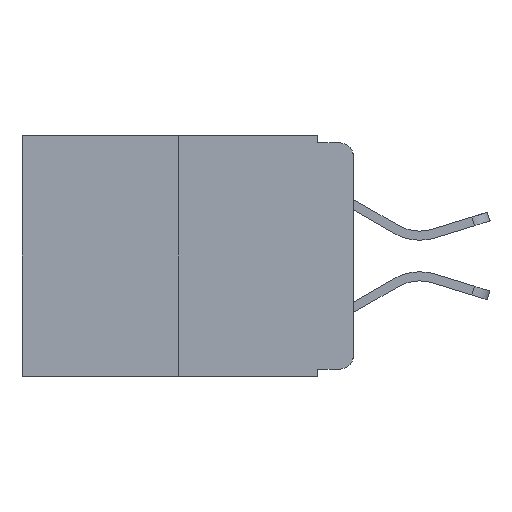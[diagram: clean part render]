
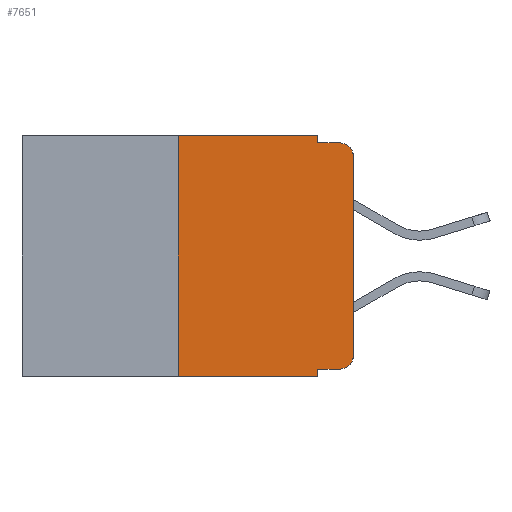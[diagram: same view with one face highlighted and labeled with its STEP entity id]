
A CAD part, left-side view. The second image highlights one B-rep face of the part: STEP entity #7651.
In plain terms, the highlighted planar face has unit normal (-1, 0, 0).
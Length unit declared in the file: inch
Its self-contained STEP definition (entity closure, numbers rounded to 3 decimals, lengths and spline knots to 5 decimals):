
#76 = CIRCLE ( 'NONE', #13283, 0.02 ) ;
#86 = ORIENTED_EDGE ( 'NONE', *, *, #2032, .F. ) ;
#299 = ORIENTED_EDGE ( 'NONE', *, *, #17580, .F. ) ;
#850 = DIRECTION ( 'NONE',  ( 1., 0., 0. ) ) ;
#975 = CARTESIAN_POINT ( 'NONE',  ( 0., 0.02, -0.03 ) ) ;
#1008 = EDGE_CURVE ( 'NONE', #21379, #19777, #14824, .T. ) ;
#1170 = VECTOR ( 'NONE', #16468, 39.37008 ) ;
#1306 = EDGE_CURVE ( 'NONE', #8760, #17799, #76, .T. ) ;
#1410 = CARTESIAN_POINT ( 'NONE',  ( 0., 0., 0. ) ) ;
#1425 = DIRECTION ( 'NONE',  ( 0., -1., 0. ) ) ;
#2007 = VECTOR ( 'NONE', #11165, 39.37008 ) ;
#2032 = EDGE_CURVE ( 'NONE', #8149, #3900, #17525, .T. ) ;
#2465 = CIRCLE ( 'NONE', #16862, 0.02 ) ;
#2495 = ORIENTED_EDGE ( 'NONE', *, *, #9484, .T. ) ;
#2614 = VERTEX_POINT ( 'NONE', #10916 ) ;
#2711 = DIRECTION ( 'NONE',  ( 0., 0., -1. ) ) ;
#3086 = FACE_OUTER_BOUND ( 'NONE', #14970, .T. ) ;
#3099 = VERTEX_POINT ( 'NONE', #3815 ) ;
#3127 = VECTOR ( 'NONE', #1425, 39.37008 ) ;
#3337 = VERTEX_POINT ( 'NONE', #9422 ) ;
#3755 = DIRECTION ( 'NONE',  ( 0., -1., 0. ) ) ;
#3815 = CARTESIAN_POINT ( 'NONE',  ( 0., 0.051, 0. ) ) ;
#3900 = VERTEX_POINT ( 'NONE', #13992 ) ;
#4194 = CARTESIAN_POINT ( 'NONE',  ( 0., 0.02, -0.333 ) ) ;
#4397 = VECTOR ( 'NONE', #12512, 39.37008 ) ;
#4543 = AXIS2_PLACEMENT_3D ( 'NONE', #11037, #850, #12675 ) ;
#4581 = CARTESIAN_POINT ( 'NONE',  ( 0., 0.051, -0.01 ) ) ;
#4670 = VERTEX_POINT ( 'NONE', #20590 ) ;
#4853 = DIRECTION ( 'NONE',  ( 0., 0., 1. ) ) ;
#5037 = CARTESIAN_POINT ( 'NONE',  ( 0., 0.25, 0. ) ) ;
#5074 = ORIENTED_EDGE ( 'NONE', *, *, #6944, .T. ) ;
#5251 = VECTOR ( 'NONE', #4853, 39.37008 ) ;
#5361 = CARTESIAN_POINT ( 'NONE',  ( 0., 0.051, -0.01 ) ) ;
#5389 = CARTESIAN_POINT ( 'NONE',  ( 0., 0.473, -0.343 ) ) ;
#6001 = CARTESIAN_POINT ( 'NONE',  ( 0., 0.051, 0. ) ) ;
#6297 = CARTESIAN_POINT ( 'NONE',  ( 0., 0.02, -0.313 ) ) ;
#6696 = CARTESIAN_POINT ( 'NONE',  ( 0., 0.473, 0. ) ) ;
#6736 = EDGE_CURVE ( 'NONE', #2614, #8760, #16357, .T. ) ;
#6944 = EDGE_CURVE ( 'NONE', #8149, #4670, #20298, .T. ) ;
#7066 = DIRECTION ( 'NONE',  ( -1., 0., 0. ) ) ;
#7651 = ADVANCED_FACE ( 'NONE', ( #3086 ), #17428, .F. ) ;
#7704 = EDGE_CURVE ( 'NONE', #2614, #4670, #11034, .T. ) ;
#8149 = VERTEX_POINT ( 'NONE', #12315 ) ;
#8176 = CARTESIAN_POINT ( 'NONE',  ( 0., 0.02, -0.01 ) ) ;
#8419 = EDGE_CURVE ( 'NONE', #3900, #3099, #14533, .T. ) ;
#8760 = VERTEX_POINT ( 'NONE', #4194 ) ;
#8970 = ORIENTED_EDGE ( 'NONE', *, *, #7704, .F. ) ;
#9360 = ORIENTED_EDGE ( 'NONE', *, *, #8419, .F. ) ;
#9422 = CARTESIAN_POINT ( 'NONE',  ( 0., 0., -0.03 ) ) ;
#9449 = LINE ( 'NONE', #6001, #17555 ) ;
#9484 = EDGE_CURVE ( 'NONE', #3337, #19777, #2465, .T. ) ;
#9651 = ORIENTED_EDGE ( 'NONE', *, *, #1306, .T. ) ;
#9728 = DIRECTION ( 'NONE',  ( 0., 0., -1. ) ) ;
#10584 = ORIENTED_EDGE ( 'NONE', *, *, #6736, .T. ) ;
#10916 = CARTESIAN_POINT ( 'NONE',  ( 0., 0.051, -0.333 ) ) ;
#11034 = LINE ( 'NONE', #11102, #2007 ) ;
#11037 = CARTESIAN_POINT ( 'NONE',  ( 0., 0.473, 0. ) ) ;
#11102 = CARTESIAN_POINT ( 'NONE',  ( 0., 0.051, 0. ) ) ;
#11165 = DIRECTION ( 'NONE',  ( 0., 0., -1. ) ) ;
#12315 = CARTESIAN_POINT ( 'NONE',  ( 0., 0.25, -0.343 ) ) ;
#12512 = DIRECTION ( 'NONE',  ( 0., 0., 1. ) ) ;
#12675 = DIRECTION ( 'NONE',  ( 0., 0., -1. ) ) ;
#12795 = DIRECTION ( 'NONE',  ( -1., 0., 0. ) ) ;
#13194 = CARTESIAN_POINT ( 'NONE',  ( 0., 0.051, -0.333 ) ) ;
#13283 = AXIS2_PLACEMENT_3D ( 'NONE', #6297, #7066, #9728 ) ;
#13727 = EDGE_CURVE ( 'NONE', #17799, #3337, #18314, .T. ) ;
#13992 = CARTESIAN_POINT ( 'NONE',  ( 0., 0.25, 0. ) ) ;
#14533 = LINE ( 'NONE', #6696, #1170 ) ;
#14824 = LINE ( 'NONE', #5361, #19039 ) ;
#14970 = EDGE_LOOP ( 'NONE', ( #17075, #2495, #20543, #299, #9360, #86, #5074, #8970, #10584, #9651 ) ) ;
#14977 = DIRECTION ( 'NONE',  ( 0., -1., 0. ) ) ;
#16098 = VECTOR ( 'NONE', #3755, 39.37008 ) ;
#16357 = LINE ( 'NONE', #13194, #3127 ) ;
#16468 = DIRECTION ( 'NONE',  ( 0., -1., 0. ) ) ;
#16862 = AXIS2_PLACEMENT_3D ( 'NONE', #975, #12795, #2711 ) ;
#17075 = ORIENTED_EDGE ( 'NONE', *, *, #13727, .T. ) ;
#17428 = PLANE ( 'NONE',  #4543 ) ;
#17479 = DIRECTION ( 'NONE',  ( 0., 0., -1. ) ) ;
#17525 = LINE ( 'NONE', #5037, #4397 ) ;
#17555 = VECTOR ( 'NONE', #17479, 39.37008 ) ;
#17580 = EDGE_CURVE ( 'NONE', #3099, #21379, #9449, .T. ) ;
#17799 = VERTEX_POINT ( 'NONE', #18017 ) ;
#18017 = CARTESIAN_POINT ( 'NONE',  ( 0., 0., -0.313 ) ) ;
#18314 = LINE ( 'NONE', #1410, #5251 ) ;
#19039 = VECTOR ( 'NONE', #14977, 39.37008 ) ;
#19777 = VERTEX_POINT ( 'NONE', #8176 ) ;
#20298 = LINE ( 'NONE', #5389, #16098 ) ;
#20543 = ORIENTED_EDGE ( 'NONE', *, *, #1008, .F. ) ;
#20590 = CARTESIAN_POINT ( 'NONE',  ( 0., 0.051, -0.343 ) ) ;
#21379 = VERTEX_POINT ( 'NONE', #4581 ) ;
